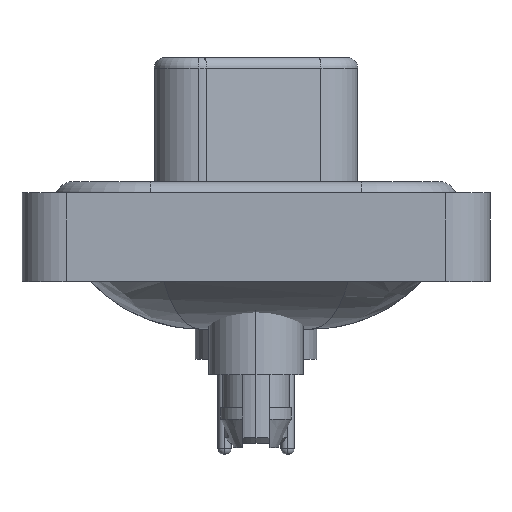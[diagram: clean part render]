
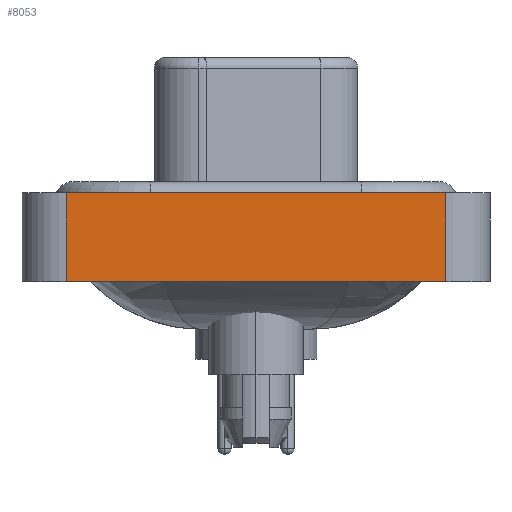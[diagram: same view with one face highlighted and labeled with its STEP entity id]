
A CAD part, left-side view. The second image highlights one B-rep face of the part: STEP entity #8053.
In plain terms, the highlighted planar face has unit normal (-1, 0, 0).
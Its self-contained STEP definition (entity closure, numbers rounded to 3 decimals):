
#78 = EDGE_CURVE ( 'NONE', #16552, #16697, #3086, .T. ) ;
#206 = CARTESIAN_POINT ( 'NONE',  ( -7.35, -8.55, -3.6 ) ) ;
#711 = CARTESIAN_POINT ( 'NONE',  ( -7.35, -8.55, -3.6 ) ) ;
#1730 = CARTESIAN_POINT ( 'NONE',  ( -7.35, -8.55, 0.4 ) ) ;
#1852 = DIRECTION ( 'NONE',  ( 0., -1., 0. ) ) ;
#2422 = EDGE_CURVE ( 'NONE', #16697, #14755, #9540, .T. ) ;
#3086 = LINE ( 'NONE', #4934, #12372 ) ;
#3130 = ORIENTED_EDGE ( 'NONE', *, *, #2422, .T. ) ;
#3540 = ORIENTED_EDGE ( 'NONE', *, *, #8271, .F. ) ;
#3801 = DIRECTION ( 'NONE',  ( 0., 0., 1. ) ) ;
#4191 = VERTEX_POINT ( 'NONE', #10888 ) ;
#4934 = CARTESIAN_POINT ( 'NONE',  ( -7.35, -8.55, -3.6 ) ) ;
#6025 = DIRECTION ( 'NONE',  ( 0., 0., 1. ) ) ;
#6401 = DIRECTION ( 'NONE',  ( 0., 0., 1. ) ) ;
#7984 = VECTOR ( 'NONE', #3801, 1000. ) ;
#8053 = ADVANCED_FACE ( 'NONE', ( #16653 ), #15136, .T. ) ;
#8271 = EDGE_CURVE ( 'NONE', #16552, #4191, #17877, .T. ) ;
#9355 = CARTESIAN_POINT ( 'NONE',  ( -7.35, 8.55, -3.6 ) ) ;
#9540 = LINE ( 'NONE', #206, #7984 ) ;
#9837 = CARTESIAN_POINT ( 'NONE',  ( -7.35, -8.55, -3.6 ) ) ;
#10888 = CARTESIAN_POINT ( 'NONE',  ( -7.35, 8.55, 0.4 ) ) ;
#11073 = VECTOR ( 'NONE', #6025, 1000. ) ;
#11867 = VECTOR ( 'NONE', #1852, 1000. ) ;
#12372 = VECTOR ( 'NONE', #20801, 1000. ) ;
#13425 = EDGE_LOOP ( 'NONE', ( #3130, #19055, #3540, #16337 ) ) ;
#13808 = LINE ( 'NONE', #1730, #11867 ) ;
#14287 = CARTESIAN_POINT ( 'NONE',  ( -7.35, 8.55, -3.6 ) ) ;
#14755 = VERTEX_POINT ( 'NONE', #21016 ) ;
#15136 = PLANE ( 'NONE',  #18034 ) ;
#16337 = ORIENTED_EDGE ( 'NONE', *, *, #78, .T. ) ;
#16552 = VERTEX_POINT ( 'NONE', #14287 ) ;
#16653 = FACE_OUTER_BOUND ( 'NONE', #13425, .T. ) ;
#16697 = VERTEX_POINT ( 'NONE', #711 ) ;
#17877 = LINE ( 'NONE', #9355, #11073 ) ;
#18034 = AXIS2_PLACEMENT_3D ( 'NONE', #9837, #22162, #6401 ) ;
#18219 = EDGE_CURVE ( 'NONE', #4191, #14755, #13808, .T. ) ;
#19055 = ORIENTED_EDGE ( 'NONE', *, *, #18219, .F. ) ;
#20801 = DIRECTION ( 'NONE',  ( 0., -1., 0. ) ) ;
#21016 = CARTESIAN_POINT ( 'NONE',  ( -7.35, -8.55, 0.4 ) ) ;
#22162 = DIRECTION ( 'NONE',  ( -1., 0., 0. ) ) ;
